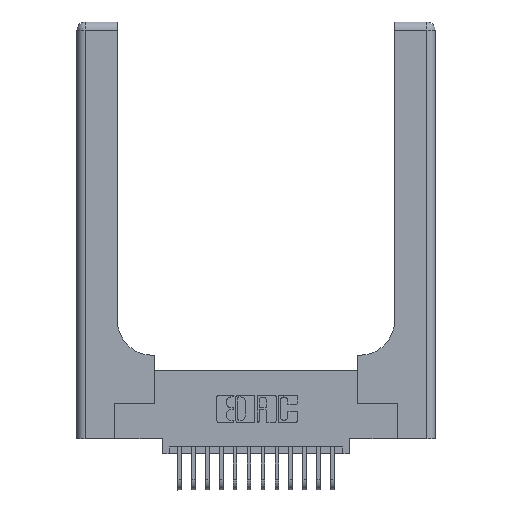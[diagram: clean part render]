
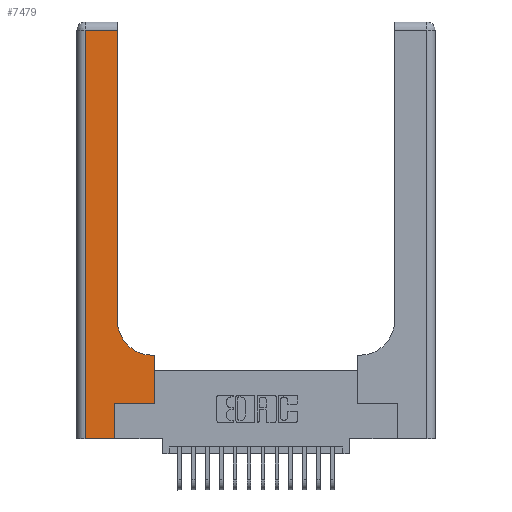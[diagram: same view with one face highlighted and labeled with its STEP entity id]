
A CAD part, top view. The second image highlights one B-rep face of the part: STEP entity #7479.
In plain terms, the highlighted planar face has unit normal (0, 0, 1).
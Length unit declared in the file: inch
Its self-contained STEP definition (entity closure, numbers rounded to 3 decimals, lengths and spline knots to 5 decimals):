
#25 = DIRECTION ( 'NONE',  ( 0., -1., 0. ) ) ;
#104 = CARTESIAN_POINT ( 'NONE',  ( 0.06, 3., 0.37 ) ) ;
#201 = CARTESIAN_POINT ( 'NONE',  ( 0., 3., 0.37 ) ) ;
#268 = DIRECTION ( 'NONE',  ( 0., 0., -1. ) ) ;
#512 = VECTOR ( 'NONE', #12782, 39.37008 ) ;
#674 = CARTESIAN_POINT ( 'NONE',  ( 0.5585, 0.25, 0.37 ) ) ;
#678 = EDGE_CURVE ( 'NONE', #11658, #3007, #6968, .T. ) ;
#1108 = AXIS2_PLACEMENT_3D ( 'NONE', #18255, #9899, #1226 ) ;
#1226 = DIRECTION ( 'NONE',  ( 1., 0., 0. ) ) ;
#1539 = CARTESIAN_POINT ( 'NONE',  ( 0.5415, 0.6, 0.37 ) ) ;
#1771 = CARTESIAN_POINT ( 'NONE',  ( 0.5585, 0.6, 0.37 ) ) ;
#2091 = ORIENTED_EDGE ( 'NONE', *, *, #13665, .T. ) ;
#2227 = VECTOR ( 'NONE', #12032, 39.37008 ) ;
#2594 = VECTOR ( 'NONE', #25, 39.37008 ) ;
#3007 = VERTEX_POINT ( 'NONE', #9566 ) ;
#3013 = VECTOR ( 'NONE', #15750, 39.37008 ) ;
#3275 = VECTOR ( 'NONE', #6635, 39.37008 ) ;
#3893 = VERTEX_POINT ( 'NONE', #8965 ) ;
#4016 = VERTEX_POINT ( 'NONE', #7817 ) ;
#4133 = VERTEX_POINT ( 'NONE', #5176 ) ;
#4483 = DIRECTION ( 'NONE',  ( 0., 1., 0. ) ) ;
#4603 = VERTEX_POINT ( 'NONE', #1539 ) ;
#4680 = PLANE ( 'NONE',  #9908 ) ;
#4898 = LINE ( 'NONE', #7120, #15692 ) ;
#5176 = CARTESIAN_POINT ( 'NONE',  ( 0.269, 0., 0.37 ) ) ;
#5901 = EDGE_LOOP ( 'NONE', ( #2091, #8444, #15034, #14137, #13083, #7060, #17017, #9436, #17761 ) ) ;
#6266 = LINE ( 'NONE', #15709, #16992 ) ;
#6635 = DIRECTION ( 'NONE',  ( 0., 1., 0. ) ) ;
#6968 = LINE ( 'NONE', #104, #2594 ) ;
#7060 = ORIENTED_EDGE ( 'NONE', *, *, #15684, .T. ) ;
#7120 = CARTESIAN_POINT ( 'NONE',  ( 0.269, 0., 0.37 ) ) ;
#7161 = LINE ( 'NONE', #13634, #3275 ) ;
#7378 = EDGE_CURVE ( 'NONE', #14825, #16319, #6266, .T. ) ;
#7479 = ADVANCED_FACE ( 'NONE', ( #16549 ), #4680, .F. ) ;
#7817 = CARTESIAN_POINT ( 'NONE',  ( 0.2915, 0.85, 0.37 ) ) ;
#7832 = LINE ( 'NONE', #8478, #512 ) ;
#7974 = CARTESIAN_POINT ( 'NONE',  ( 0.2915, 0.6, 0.37 ) ) ;
#8444 = ORIENTED_EDGE ( 'NONE', *, *, #9979, .T. ) ;
#8478 = CARTESIAN_POINT ( 'NONE',  ( 0., 0., 0.37 ) ) ;
#8965 = CARTESIAN_POINT ( 'NONE',  ( 0.2915, 2.94, 0.37 ) ) ;
#9362 = DIRECTION ( 'NONE',  ( -1., 0., 0. ) ) ;
#9436 = ORIENTED_EDGE ( 'NONE', *, *, #10699, .T. ) ;
#9566 = CARTESIAN_POINT ( 'NONE',  ( 0.06, 0., 0.37 ) ) ;
#9899 = DIRECTION ( 'NONE',  ( 0., 0., -1. ) ) ;
#9908 = AXIS2_PLACEMENT_3D ( 'NONE', #201, #268, #10399 ) ;
#9912 = VECTOR ( 'NONE', #9362, 39.37008 ) ;
#9979 = EDGE_CURVE ( 'NONE', #3893, #11658, #17341, .T. ) ;
#9994 = DIRECTION ( 'NONE',  ( 0., 1., 0. ) ) ;
#10399 = DIRECTION ( 'NONE',  ( -1., 0., 0. ) ) ;
#10689 = CARTESIAN_POINT ( 'NONE',  ( 0.269, 0.25, 0.37 ) ) ;
#10699 = EDGE_CURVE ( 'NONE', #16319, #4603, #17345, .T. ) ;
#11559 = CARTESIAN_POINT ( 'NONE',  ( 0.269, 0.25, 0.37 ) ) ;
#11658 = VERTEX_POINT ( 'NONE', #17362 ) ;
#12032 = DIRECTION ( 'NONE',  ( -1., 0., 0. ) ) ;
#12382 = VERTEX_POINT ( 'NONE', #10689 ) ;
#12782 = DIRECTION ( 'NONE',  ( 1., 0., 0. ) ) ;
#13083 = ORIENTED_EDGE ( 'NONE', *, *, #13817, .T. ) ;
#13391 = EDGE_CURVE ( 'NONE', #4603, #4016, #15267, .T. ) ;
#13422 = EDGE_CURVE ( 'NONE', #3007, #4133, #7832, .T. ) ;
#13634 = CARTESIAN_POINT ( 'NONE',  ( 0.2915, 3., 0.37 ) ) ;
#13665 = EDGE_CURVE ( 'NONE', #4016, #3893, #7161, .T. ) ;
#13817 = EDGE_CURVE ( 'NONE', #4133, #12382, #4898, .T. ) ;
#14137 = ORIENTED_EDGE ( 'NONE', *, *, #13422, .T. ) ;
#14825 = VERTEX_POINT ( 'NONE', #674 ) ;
#14846 = CARTESIAN_POINT ( 'NONE',  ( 0., 2.94, 0.37 ) ) ;
#15034 = ORIENTED_EDGE ( 'NONE', *, *, #678, .T. ) ;
#15267 = CIRCLE ( 'NONE', #1108, 0.25 ) ;
#15684 = EDGE_CURVE ( 'NONE', #12382, #14825, #18078, .T. ) ;
#15692 = VECTOR ( 'NONE', #9994, 39.37008 ) ;
#15709 = CARTESIAN_POINT ( 'NONE',  ( 0.5585, 0.25, 0.37 ) ) ;
#15750 = DIRECTION ( 'NONE',  ( 1., 0., 0. ) ) ;
#16319 = VERTEX_POINT ( 'NONE', #1771 ) ;
#16549 = FACE_OUTER_BOUND ( 'NONE', #5901, .T. ) ;
#16992 = VECTOR ( 'NONE', #4483, 39.37008 ) ;
#17017 = ORIENTED_EDGE ( 'NONE', *, *, #7378, .T. ) ;
#17341 = LINE ( 'NONE', #14846, #2227 ) ;
#17345 = LINE ( 'NONE', #7974, #9912 ) ;
#17362 = CARTESIAN_POINT ( 'NONE',  ( 0.06, 2.94, 0.37 ) ) ;
#17761 = ORIENTED_EDGE ( 'NONE', *, *, #13391, .T. ) ;
#18078 = LINE ( 'NONE', #11559, #3013 ) ;
#18255 = CARTESIAN_POINT ( 'NONE',  ( 0.5415, 0.85, 0.37 ) ) ;
